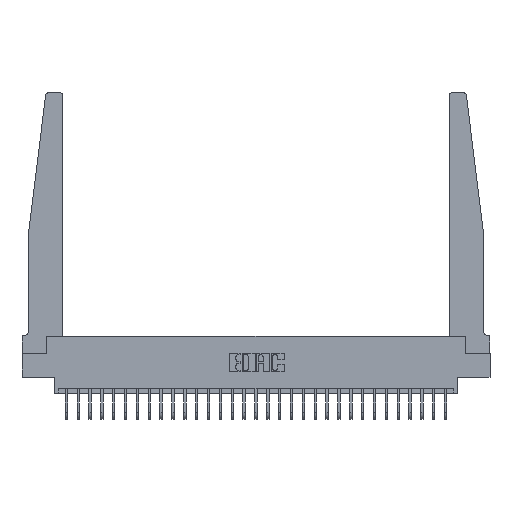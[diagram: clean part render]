
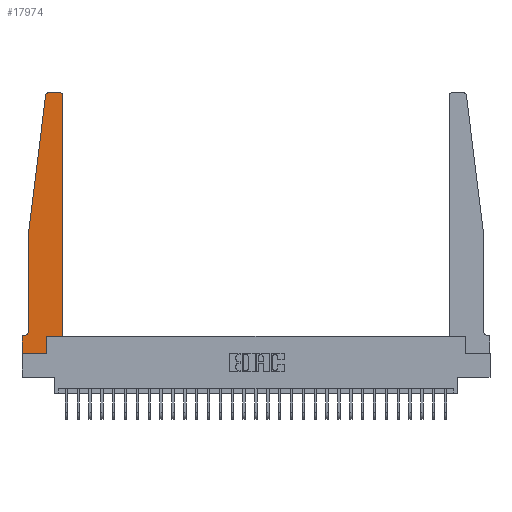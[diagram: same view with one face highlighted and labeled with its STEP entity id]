
A CAD part, top view. The second image highlights one B-rep face of the part: STEP entity #17974.
In plain terms, the highlighted planar face has unit normal (0, 0, 1).
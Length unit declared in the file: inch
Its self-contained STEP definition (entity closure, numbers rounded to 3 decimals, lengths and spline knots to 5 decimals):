
#431 = LINE ( 'NONE', #19366, #26577 ) ;
#539 = LINE ( 'NONE', #9034, #4922 ) ;
#569 = DIRECTION ( 'NONE',  ( 1., 0., 0. ) ) ;
#592 = VERTEX_POINT ( 'NONE', #10647 ) ;
#627 = LINE ( 'NONE', #2532, #11618 ) ;
#927 = DIRECTION ( 'NONE',  ( -1., 0., 0. ) ) ;
#951 = FACE_OUTER_BOUND ( 'NONE', #7826, .T. ) ;
#2253 = DIRECTION ( 'NONE',  ( 1., 0., 0. ) ) ;
#2532 = CARTESIAN_POINT ( 'NONE',  ( 0., 0., 0.37 ) ) ;
#2991 = AXIS2_PLACEMENT_3D ( 'NONE', #26089, #25551, #25953 ) ;
#3420 = VECTOR ( 'NONE', #18353, 39.37008 ) ;
#3562 = CARTESIAN_POINT ( 'NONE',  ( 0.425, 0.18, 0.37 ) ) ;
#3885 = CIRCLE ( 'NONE', #2991, 0.03 ) ;
#4220 = LINE ( 'NONE', #25216, #10904 ) ;
#4370 = CIRCLE ( 'NONE', #10074, 0.03 ) ;
#4443 = EDGE_CURVE ( 'NONE', #592, #13121, #4517, .T. ) ;
#4497 = DIRECTION ( 'NONE',  ( -1., 0., 0. ) ) ;
#4517 = LINE ( 'NONE', #12896, #12251 ) ;
#4613 = EDGE_CURVE ( 'NONE', #18511, #16460, #12324, .T. ) ;
#4805 = DIRECTION ( 'NONE',  ( 1., 0., 0. ) ) ;
#4922 = VECTOR ( 'NONE', #8897, 39.37008 ) ;
#5134 = ORIENTED_EDGE ( 'NONE', *, *, #9649, .T. ) ;
#5210 = CARTESIAN_POINT ( 'NONE',  ( 0.015, 0.1875, 0.37 ) ) ;
#6242 = ORIENTED_EDGE ( 'NONE', *, *, #4443, .T. ) ;
#6484 = EDGE_CURVE ( 'NONE', #11570, #15353, #4370, .T. ) ;
#7435 = VERTEX_POINT ( 'NONE', #19342 ) ;
#7826 = EDGE_LOOP ( 'NONE', ( #13239, #17766, #15741, #18406, #10177, #22381, #14800, #15355, #5134, #6242, #19670, #15291 ) ) ;
#8395 = VERTEX_POINT ( 'NONE', #17385 ) ;
#8897 = DIRECTION ( 'NONE',  ( 0., 1., 0. ) ) ;
#9034 = CARTESIAN_POINT ( 'NONE',  ( 0.2605, 0.18, 0.37 ) ) ;
#9147 = LINE ( 'NONE', #10951, #25481 ) ;
#9189 = CARTESIAN_POINT ( 'NONE',  ( 0., 0.1875, 0.37 ) ) ;
#9274 = EDGE_CURVE ( 'NONE', #22870, #15119, #431, .T. ) ;
#9526 = CARTESIAN_POINT ( 'NONE',  ( 0.065, 1.25, 0.37 ) ) ;
#9649 = EDGE_CURVE ( 'NONE', #15119, #592, #539, .T. ) ;
#10074 = AXIS2_PLACEMENT_3D ( 'NONE', #12971, #14890, #2253 ) ;
#10177 = ORIENTED_EDGE ( 'NONE', *, *, #19009, .T. ) ;
#10482 = CIRCLE ( 'NONE', #20144, 0.05 ) ;
#10506 = VECTOR ( 'NONE', #927, 39.37008 ) ;
#10647 = CARTESIAN_POINT ( 'NONE',  ( 0.2605, 0.18, 0.37 ) ) ;
#10830 = DIRECTION ( 'NONE',  ( 1., 0., 0. ) ) ;
#10904 = VECTOR ( 'NONE', #19445, 39.37008 ) ;
#10951 = CARTESIAN_POINT ( 'NONE',  ( 0.25, 2.75, 0.37 ) ) ;
#11470 = DIRECTION ( 'NONE',  ( 0., -1., 0. ) ) ;
#11570 = VERTEX_POINT ( 'NONE', #12566 ) ;
#11618 = VECTOR ( 'NONE', #11470, 39.37008 ) ;
#11751 = CARTESIAN_POINT ( 'NONE',  ( 0., 0., 0.37 ) ) ;
#12251 = VECTOR ( 'NONE', #10830, 39.37008 ) ;
#12263 = EDGE_CURVE ( 'NONE', #7435, #22870, #627, .T. ) ;
#12324 = LINE ( 'NONE', #22075, #3420 ) ;
#12566 = CARTESIAN_POINT ( 'NONE',  ( 0.425, 2.72, 0.37 ) ) ;
#12896 = CARTESIAN_POINT ( 'NONE',  ( 0.425, 0.18, 0.37 ) ) ;
#12971 = CARTESIAN_POINT ( 'NONE',  ( 0.395, 2.72, 0.37 ) ) ;
#13121 = VERTEX_POINT ( 'NONE', #3562 ) ;
#13239 = ORIENTED_EDGE ( 'NONE', *, *, #25085, .T. ) ;
#13438 = CARTESIAN_POINT ( 'NONE',  ( 0.065, 0.1875, 0.37 ) ) ;
#13555 = VECTOR ( 'NONE', #18774, 39.37008 ) ;
#13811 = CARTESIAN_POINT ( 'NONE',  ( 0.065, 0.2375, 0.37 ) ) ;
#14527 = CARTESIAN_POINT ( 'NONE',  ( 0.395, 2.75, 0.37 ) ) ;
#14800 = ORIENTED_EDGE ( 'NONE', *, *, #12263, .T. ) ;
#14890 = DIRECTION ( 'NONE',  ( 0., 0., 1. ) ) ;
#15119 = VERTEX_POINT ( 'NONE', #15548 ) ;
#15291 = ORIENTED_EDGE ( 'NONE', *, *, #6484, .T. ) ;
#15353 = VERTEX_POINT ( 'NONE', #14527 ) ;
#15355 = ORIENTED_EDGE ( 'NONE', *, *, #9274, .T. ) ;
#15548 = CARTESIAN_POINT ( 'NONE',  ( 0.2605, 0., 0.37 ) ) ;
#15741 = ORIENTED_EDGE ( 'NONE', *, *, #16606, .T. ) ;
#16105 = DIRECTION ( 'NONE',  ( 0., 0., -1. ) ) ;
#16300 = EDGE_CURVE ( 'NONE', #8395, #24022, #3885, .T. ) ;
#16376 = DIRECTION ( 'NONE',  ( -1., 0., 0. ) ) ;
#16460 = VERTEX_POINT ( 'NONE', #13811 ) ;
#16606 = EDGE_CURVE ( 'NONE', #24022, #18511, #4220, .T. ) ;
#17385 = CARTESIAN_POINT ( 'NONE',  ( 0.27653, 2.75, 0.37 ) ) ;
#17711 = PLANE ( 'NONE',  #26647 ) ;
#17766 = ORIENTED_EDGE ( 'NONE', *, *, #16300, .T. ) ;
#17974 = ADVANCED_FACE ( 'NONE', ( #951 ), #17711, .T. ) ;
#18230 = EDGE_CURVE ( 'NONE', #13121, #11570, #19050, .T. ) ;
#18353 = DIRECTION ( 'NONE',  ( 0., -1., 0. ) ) ;
#18406 = ORIENTED_EDGE ( 'NONE', *, *, #4613, .T. ) ;
#18511 = VERTEX_POINT ( 'NONE', #9526 ) ;
#18774 = DIRECTION ( 'NONE',  ( 0., 1., 0. ) ) ;
#19009 = EDGE_CURVE ( 'NONE', #16460, #24806, #10482, .T. ) ;
#19050 = LINE ( 'NONE', #26879, #13555 ) ;
#19342 = CARTESIAN_POINT ( 'NONE',  ( 0., 0.1875, 0.37 ) ) ;
#19366 = CARTESIAN_POINT ( 'NONE',  ( 0., 0., 0.37 ) ) ;
#19445 = DIRECTION ( 'NONE',  ( -0.122, -0.992, 0. ) ) ;
#19625 = DIRECTION ( 'NONE',  ( 0., 0., 1. ) ) ;
#19670 = ORIENTED_EDGE ( 'NONE', *, *, #18230, .T. ) ;
#19760 = EDGE_CURVE ( 'NONE', #24806, #7435, #21676, .T. ) ;
#20144 = AXIS2_PLACEMENT_3D ( 'NONE', #24444, #16105, #16376 ) ;
#21676 = LINE ( 'NONE', #13438, #10506 ) ;
#22075 = CARTESIAN_POINT ( 'NONE',  ( 0.065, 1.25, 0.37 ) ) ;
#22381 = ORIENTED_EDGE ( 'NONE', *, *, #19760, .T. ) ;
#22870 = VERTEX_POINT ( 'NONE', #11751 ) ;
#23236 = CARTESIAN_POINT ( 'NONE',  ( 0.24675, 2.72367, 0.37 ) ) ;
#24022 = VERTEX_POINT ( 'NONE', #23236 ) ;
#24444 = CARTESIAN_POINT ( 'NONE',  ( 0.015, 0.2375, 0.37 ) ) ;
#24806 = VERTEX_POINT ( 'NONE', #5210 ) ;
#25085 = EDGE_CURVE ( 'NONE', #15353, #8395, #9147, .T. ) ;
#25216 = CARTESIAN_POINT ( 'NONE',  ( 0.065, 1.25, 0.37 ) ) ;
#25481 = VECTOR ( 'NONE', #4497, 39.37008 ) ;
#25551 = DIRECTION ( 'NONE',  ( 0., 0., 1. ) ) ;
#25953 = DIRECTION ( 'NONE',  ( 1., 0., 0. ) ) ;
#26089 = CARTESIAN_POINT ( 'NONE',  ( 0.27653, 2.72, 0.37 ) ) ;
#26577 = VECTOR ( 'NONE', #569, 39.37008 ) ;
#26647 = AXIS2_PLACEMENT_3D ( 'NONE', #9189, #19625, #4805 ) ;
#26879 = CARTESIAN_POINT ( 'NONE',  ( 0.425, 0.18, 0.37 ) ) ;
